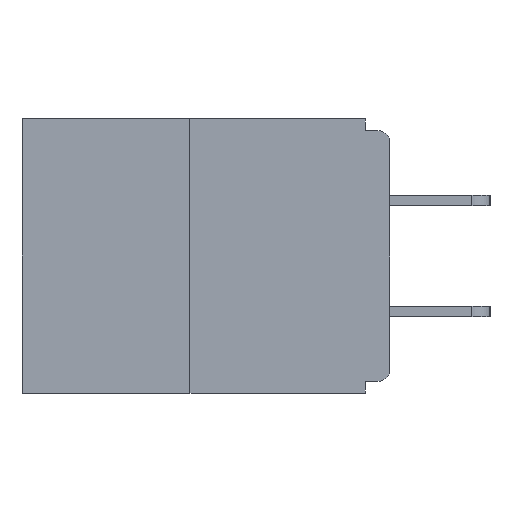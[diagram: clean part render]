
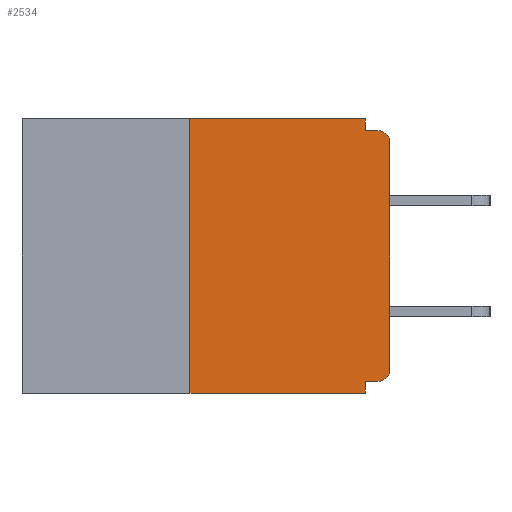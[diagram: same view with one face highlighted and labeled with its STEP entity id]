
A CAD part, left-side view. The second image highlights one B-rep face of the part: STEP entity #2534.
In plain terms, the highlighted planar face has unit normal (-1, 0, 0).
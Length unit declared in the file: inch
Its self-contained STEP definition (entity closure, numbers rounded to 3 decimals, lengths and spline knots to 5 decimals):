
#314 = EDGE_CURVE ( 'NONE', #15935, #4695, #17666, .T. ) ;
#341 = CARTESIAN_POINT ( 'NONE',  ( 0., 0.031, -0.343 ) ) ;
#900 = DIRECTION ( 'NONE',  ( 0., 1., 0. ) ) ;
#912 = ORIENTED_EDGE ( 'NONE', *, *, #14830, .T. ) ;
#978 = EDGE_CURVE ( 'NONE', #7098, #15935, #1139, .T. ) ;
#1139 = CIRCLE ( 'NONE', #18644, 0.015 ) ;
#2117 = LINE ( 'NONE', #17518, #3931 ) ;
#2121 = CARTESIAN_POINT ( 'NONE',  ( 0., 0.25, 0. ) ) ;
#2148 = EDGE_CURVE ( 'NONE', #19845, #19890, #2117, .T. ) ;
#2153 = EDGE_CURVE ( 'NONE', #7098, #10425, #5999, .T. ) ;
#2534 = ADVANCED_FACE ( 'NONE', ( #11712 ), #3752, .F. ) ;
#2641 = VERTEX_POINT ( 'NONE', #20967 ) ;
#3432 = VECTOR ( 'NONE', #900, 39.37008 ) ;
#3598 = DIRECTION ( 'NONE',  ( 0., -1., 0. ) ) ;
#3752 = PLANE ( 'NONE',  #5666 ) ;
#3881 = CARTESIAN_POINT ( 'NONE',  ( 0., 0.25, 0. ) ) ;
#3931 = VECTOR ( 'NONE', #9011, 39.37008 ) ;
#4242 = ORIENTED_EDGE ( 'NONE', *, *, #14042, .F. ) ;
#4415 = VECTOR ( 'NONE', #3598, 39.37008 ) ;
#4680 = ORIENTED_EDGE ( 'NONE', *, *, #17443, .F. ) ;
#4695 = VERTEX_POINT ( 'NONE', #19179 ) ;
#5217 = DIRECTION ( 'NONE',  ( -1., 0., 0. ) ) ;
#5396 = DIRECTION ( 'NONE',  ( 1., 0., 0. ) ) ;
#5666 = AXIS2_PLACEMENT_3D ( 'NONE', #15390, #5396, #17047 ) ;
#5999 = LINE ( 'NONE', #10836, #3432 ) ;
#6123 = CARTESIAN_POINT ( 'NONE',  ( 0., 0.015, -0.313 ) ) ;
#6400 = CARTESIAN_POINT ( 'NONE',  ( 0., 0.015, -0.328 ) ) ;
#6553 = DIRECTION ( 'NONE',  ( 0., -1., 0. ) ) ;
#6645 = VERTEX_POINT ( 'NONE', #7482 ) ;
#6948 = CARTESIAN_POINT ( 'NONE',  ( 0., 0.031, 0. ) ) ;
#7098 = VERTEX_POINT ( 'NONE', #6400 ) ;
#7482 = CARTESIAN_POINT ( 'NONE',  ( 0., 0.25, -0.343 ) ) ;
#7547 = ORIENTED_EDGE ( 'NONE', *, *, #978, .T. ) ;
#7954 = CARTESIAN_POINT ( 'NONE',  ( 0., 0.031, -0.328 ) ) ;
#8043 = DIRECTION ( 'NONE',  ( 0., 0., -1. ) ) ;
#8048 = CARTESIAN_POINT ( 'NONE',  ( 0., 0., -0.313 ) ) ;
#8347 = AXIS2_PLACEMENT_3D ( 'NONE', #9487, #5217, #16854 ) ;
#8661 = VECTOR ( 'NONE', #17004, 39.37008 ) ;
#8814 = DIRECTION ( 'NONE',  ( 0., 0., -1. ) ) ;
#9011 = DIRECTION ( 'NONE',  ( 0., -1., 0. ) ) ;
#9487 = CARTESIAN_POINT ( 'NONE',  ( 0., 0.015, -0.03 ) ) ;
#9621 = VERTEX_POINT ( 'NONE', #12400 ) ;
#10425 = VERTEX_POINT ( 'NONE', #7954 ) ;
#10748 = ORIENTED_EDGE ( 'NONE', *, *, #17509, .F. ) ;
#10789 = VECTOR ( 'NONE', #6553, 39.37008 ) ;
#10836 = CARTESIAN_POINT ( 'NONE',  ( 0., 0., -0.328 ) ) ;
#11012 = CARTESIAN_POINT ( 'NONE',  ( 0., 0.031, 0. ) ) ;
#11301 = VECTOR ( 'NONE', #8814, 39.37008 ) ;
#11358 = DIRECTION ( 'NONE',  ( 0., 0., 1. ) ) ;
#11712 = FACE_OUTER_BOUND ( 'NONE', #12207, .T. ) ;
#11953 = EDGE_CURVE ( 'NONE', #4695, #9621, #18033, .T. ) ;
#11960 = EDGE_CURVE ( 'NONE', #19890, #2641, #13085, .T. ) ;
#12094 = CARTESIAN_POINT ( 'NONE',  ( 0., 0.46, -0.343 ) ) ;
#12207 = EDGE_LOOP ( 'NONE', ( #16989, #4242, #912, #10748, #19817, #7547, #17736, #21463, #4680, #15443 ) ) ;
#12400 = CARTESIAN_POINT ( 'NONE',  ( 0., 0.015, -0.015 ) ) ;
#12744 = CARTESIAN_POINT ( 'NONE',  ( 0., 0.031, -0.343 ) ) ;
#13085 = LINE ( 'NONE', #6948, #8661 ) ;
#14042 = EDGE_CURVE ( 'NONE', #6645, #19845, #20369, .T. ) ;
#14414 = VERTEX_POINT ( 'NONE', #12744 ) ;
#14516 = CARTESIAN_POINT ( 'NONE',  ( 0., 0., 0. ) ) ;
#14830 = EDGE_CURVE ( 'NONE', #6645, #14414, #17688, .T. ) ;
#15390 = CARTESIAN_POINT ( 'NONE',  ( 0., 0.46, 0. ) ) ;
#15443 = ORIENTED_EDGE ( 'NONE', *, *, #11960, .F. ) ;
#15935 = VERTEX_POINT ( 'NONE', #8048 ) ;
#16047 = DIRECTION ( 'NONE',  ( -1., 0., 0. ) ) ;
#16265 = LINE ( 'NONE', #341, #11301 ) ;
#16854 = DIRECTION ( 'NONE',  ( 0., 0., -1. ) ) ;
#16989 = ORIENTED_EDGE ( 'NONE', *, *, #2148, .F. ) ;
#17004 = DIRECTION ( 'NONE',  ( 0., 0., -1. ) ) ;
#17047 = DIRECTION ( 'NONE',  ( 0., 0., -1. ) ) ;
#17443 = EDGE_CURVE ( 'NONE', #2641, #9621, #20211, .T. ) ;
#17509 = EDGE_CURVE ( 'NONE', #10425, #14414, #16265, .T. ) ;
#17518 = CARTESIAN_POINT ( 'NONE',  ( 0., 0.46, 0. ) ) ;
#17666 = LINE ( 'NONE', #14516, #21109 ) ;
#17688 = LINE ( 'NONE', #12094, #4415 ) ;
#17736 = ORIENTED_EDGE ( 'NONE', *, *, #314, .T. ) ;
#18033 = CIRCLE ( 'NONE', #8347, 0.015 ) ;
#18222 = CARTESIAN_POINT ( 'NONE',  ( 0., 0., -0.015 ) ) ;
#18644 = AXIS2_PLACEMENT_3D ( 'NONE', #6123, #16047, #8043 ) ;
#19179 = CARTESIAN_POINT ( 'NONE',  ( 0., 0., -0.03 ) ) ;
#19817 = ORIENTED_EDGE ( 'NONE', *, *, #2153, .F. ) ;
#19845 = VERTEX_POINT ( 'NONE', #3881 ) ;
#19890 = VERTEX_POINT ( 'NONE', #11012 ) ;
#20211 = LINE ( 'NONE', #18222, #10789 ) ;
#20362 = DIRECTION ( 'NONE',  ( 0., 0., 1. ) ) ;
#20369 = LINE ( 'NONE', #2121, #21394 ) ;
#20967 = CARTESIAN_POINT ( 'NONE',  ( 0., 0.031, -0.015 ) ) ;
#21109 = VECTOR ( 'NONE', #11358, 39.37008 ) ;
#21394 = VECTOR ( 'NONE', #20362, 39.37008 ) ;
#21463 = ORIENTED_EDGE ( 'NONE', *, *, #11953, .T. ) ;
